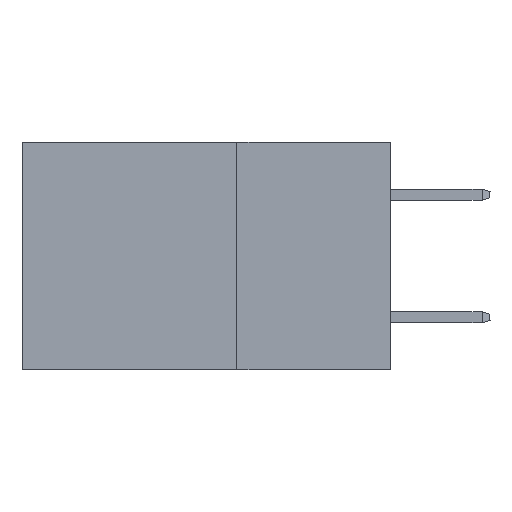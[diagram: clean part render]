
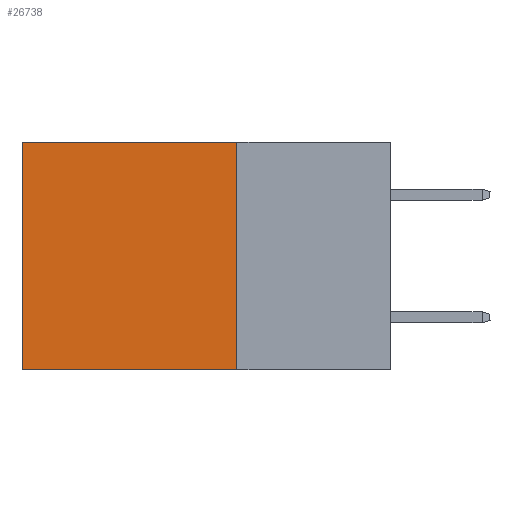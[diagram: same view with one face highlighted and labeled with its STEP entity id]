
A CAD part, left-side view. The second image highlights one B-rep face of the part: STEP entity #26738.
In plain terms, the highlighted planar face has unit normal (-1, 0, 0).
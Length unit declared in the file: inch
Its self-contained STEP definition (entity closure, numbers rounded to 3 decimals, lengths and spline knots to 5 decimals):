
#307 = VECTOR ( 'NONE', #29073, 39.37008 ) ;
#1430 = CARTESIAN_POINT ( 'NONE',  ( 0.2875, 0.6, 0. ) ) ;
#2877 = LINE ( 'NONE', #18781, #9449 ) ;
#4847 = CARTESIAN_POINT ( 'NONE',  ( 0.2875, 0.25, 0. ) ) ;
#6706 = EDGE_CURVE ( 'NONE', #33389, #26455, #22516, .T. ) ;
#6815 = DIRECTION ( 'NONE',  ( 0., 0., -1. ) ) ;
#6876 = VERTEX_POINT ( 'NONE', #35113 ) ;
#7417 = EDGE_LOOP ( 'NONE', ( #29064, #14402, #34998, #14770 ) ) ;
#7679 = DIRECTION ( 'NONE',  ( 0., 0., -1. ) ) ;
#9449 = VECTOR ( 'NONE', #10530, 39.37008 ) ;
#10530 = DIRECTION ( 'NONE',  ( 0., 1., 0. ) ) ;
#13188 = LINE ( 'NONE', #31683, #28618 ) ;
#13723 = VERTEX_POINT ( 'NONE', #1430 ) ;
#14402 = ORIENTED_EDGE ( 'NONE', *, *, #6706, .F. ) ;
#14770 = ORIENTED_EDGE ( 'NONE', *, *, #34568, .T. ) ;
#15075 = CARTESIAN_POINT ( 'NONE',  ( 0.2875, 0.6, 0. ) ) ;
#16679 = CARTESIAN_POINT ( 'NONE',  ( 0.2875, 0.25, -0.37 ) ) ;
#18715 = FACE_OUTER_BOUND ( 'NONE', #7417, .T. ) ;
#18781 = CARTESIAN_POINT ( 'NONE',  ( 0.2875, 0.25, 0. ) ) ;
#19788 = LINE ( 'NONE', #15075, #34108 ) ;
#21476 = PLANE ( 'NONE',  #22746 ) ;
#22347 = EDGE_CURVE ( 'NONE', #6876, #33389, #13188, .T. ) ;
#22516 = LINE ( 'NONE', #26384, #307 ) ;
#22746 = AXIS2_PLACEMENT_3D ( 'NONE', #4847, #24233, #7679 ) ;
#24233 = DIRECTION ( 'NONE',  ( 1., 0., 0. ) ) ;
#26384 = CARTESIAN_POINT ( 'NONE',  ( 0.2875, 0.25, -0.37 ) ) ;
#26455 = VERTEX_POINT ( 'NONE', #33845 ) ;
#26738 = ADVANCED_FACE ( 'NONE', ( #18715 ), #21476, .F. ) ;
#28618 = VECTOR ( 'NONE', #29010, 39.37008 ) ;
#29010 = DIRECTION ( 'NONE',  ( 0., 0., -1. ) ) ;
#29064 = ORIENTED_EDGE ( 'NONE', *, *, #34056, .T. ) ;
#29073 = DIRECTION ( 'NONE',  ( 0., 1., 0. ) ) ;
#31683 = CARTESIAN_POINT ( 'NONE',  ( 0.2875, 0.25, 0. ) ) ;
#33389 = VERTEX_POINT ( 'NONE', #16679 ) ;
#33845 = CARTESIAN_POINT ( 'NONE',  ( 0.2875, 0.6, -0.37 ) ) ;
#34056 = EDGE_CURVE ( 'NONE', #13723, #26455, #19788, .T. ) ;
#34108 = VECTOR ( 'NONE', #6815, 39.37008 ) ;
#34568 = EDGE_CURVE ( 'NONE', #6876, #13723, #2877, .T. ) ;
#34998 = ORIENTED_EDGE ( 'NONE', *, *, #22347, .F. ) ;
#35113 = CARTESIAN_POINT ( 'NONE',  ( 0.2875, 0.25, 0. ) ) ;
